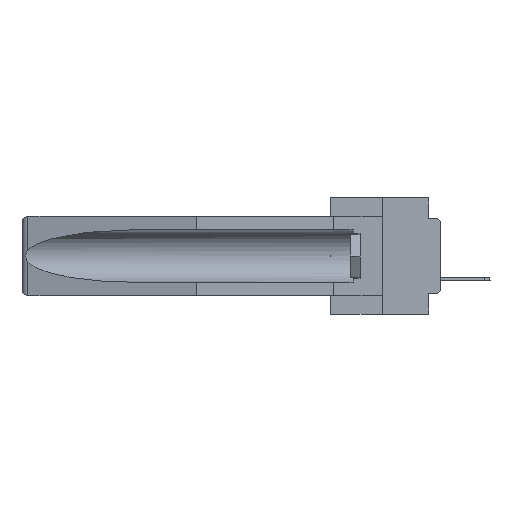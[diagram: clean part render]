
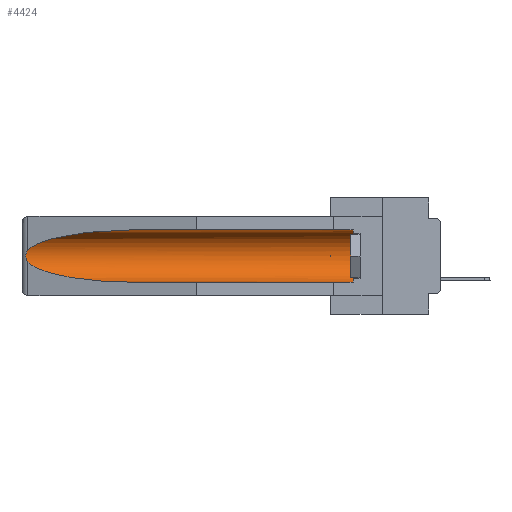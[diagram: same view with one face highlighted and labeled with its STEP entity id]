
A CAD part, left-side view. The second image highlights one B-rep face of the part: STEP entity #4424.
In plain terms, the highlighted cylindrical face has radius 2.857 mm (diameter 5.715 mm), a partial arc.
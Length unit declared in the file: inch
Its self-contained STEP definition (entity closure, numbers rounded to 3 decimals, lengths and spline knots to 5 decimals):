
#463 = EDGE_CURVE ( 'NONE', #9557, #4743, #7884, .T. ) ;
#1396 = CARTESIAN_POINT ( 'NONE',  ( 0.155, -0.30754, -0.284 ) ) ;
#2283 = CARTESIAN_POINT ( 'NONE',  ( 0.2673, 1.53269, -0.17917 ) ) ;
#2791 = DIRECTION ( 'NONE',  ( 0., 1., 0. ) ) ;
#3652 = VECTOR ( 'NONE', #22807, 39.37008 ) ;
#4424 = ADVANCED_FACE ( 'NONE', ( #13636 ), #19963, .F. ) ;
#4743 = VERTEX_POINT ( 'NONE', #22501 ) ;
#5068 = CARTESIAN_POINT ( 'NONE',  ( 0.26654, 1.53092, -0.15636 ) ) ;
#5445 = CIRCLE ( 'NONE', #13716, 0.1125 ) ;
#6375 = EDGE_CURVE ( 'NONE', #7409, #33984, #18339, .T. ) ;
#6435 = CARTESIAN_POINT ( 'NONE',  ( 0.155, 0.126, -0.284 ) ) ;
#7055 = CARTESIAN_POINT ( 'NONE',  ( 0.26537, 1.52718, -0.14972 ) ) ;
#7095 = DIRECTION ( 'NONE',  ( 0., 1., 0. ) ) ;
#7409 = VERTEX_POINT ( 'NONE', #22976 ) ;
#7884 =( BOUNDED_CURVE ( )  B_SPLINE_CURVE ( 3, ( #34929, #10754, #35115, #38264 ),
 .UNSPECIFIED., .F., .F. ) 
 B_SPLINE_CURVE_WITH_KNOTS ( ( 4, 4 ),
 ( 0.1948, 1.5708 ),
 .UNSPECIFIED. ) 
 CURVE ( )  GEOMETRIC_REPRESENTATION_ITEM ( )  RATIONAL_B_SPLINE_CURVE ( ( 1., 0.848, 0.848, 1. ) ) 
 REPRESENTATION_ITEM ( '' )  );
#8369 = CARTESIAN_POINT ( 'NONE',  ( 0.155, -0.30754, -0.059 ) ) ;
#8754 = VECTOR ( 'NONE', #2791, 39.37008 ) ;
#9080 = ORIENTED_EDGE ( 'NONE', *, *, #28041, .T. ) ;
#9557 = VERTEX_POINT ( 'NONE', #36418 ) ;
#10074 = CARTESIAN_POINT ( 'NONE',  ( 0.25451, 1.48313, -0.09465 ) ) ;
#10754 = CARTESIAN_POINT ( 'NONE',  ( 0.25451, 1.48313, -0.24835 ) ) ;
#11154 = EDGE_CURVE ( 'NONE', #33984, #9557, #23094, .T. ) ;
#11438 = CARTESIAN_POINT ( 'NONE',  ( 0.26597, 1.5296, -0.19026 ) ) ;
#12276 = CARTESIAN_POINT ( 'NONE',  ( 0.21114, 1.30732, -0.059 ) ) ;
#13636 = FACE_OUTER_BOUND ( 'NONE', #32733, .T. ) ;
#13716 = AXIS2_PLACEMENT_3D ( 'NONE', #17679, #20637, #29754 ) ;
#15459 = ORIENTED_EDGE ( 'NONE', *, *, #29558, .F. ) ;
#16698 = CARTESIAN_POINT ( 'NONE',  ( 0.155, 0.126, -0.059 ) ) ;
#17679 = CARTESIAN_POINT ( 'NONE',  ( 0.155, 0.126, -0.1715 ) ) ;
#18339 =( BOUNDED_CURVE ( )  B_SPLINE_CURVE ( 3, ( #37214, #12276, #10074, #27896 ),
 .UNSPECIFIED., .F., .F. ) 
 B_SPLINE_CURVE_WITH_KNOTS ( ( 4, 4 ),
 ( 4.71239, 6.08839 ),
 .UNSPECIFIED. ) 
 CURVE ( )  GEOMETRIC_REPRESENTATION_ITEM ( )  RATIONAL_B_SPLINE_CURVE ( ( 1., 0.848, 0.848, 1. ) ) 
 REPRESENTATION_ITEM ( '' )  );
#19208 = CARTESIAN_POINT ( 'NONE',  ( 0.155, -0.30754, -0.1715 ) ) ;
#19449 = LINE ( 'NONE', #1396, #3652 ) ;
#19963 = CYLINDRICAL_SURFACE ( 'NONE', #31102, 0.1125 ) ;
#20637 = DIRECTION ( 'NONE',  ( 0., -1., 0. ) ) ;
#22408 = ORIENTED_EDGE ( 'NONE', *, *, #463, .T. ) ;
#22501 = CARTESIAN_POINT ( 'NONE',  ( 0.155, 1.07973, -0.284 ) ) ;
#22736 = CARTESIAN_POINT ( 'NONE',  ( 0.2675, 1.53308, -0.16763 ) ) ;
#22807 = DIRECTION ( 'NONE',  ( 0., 1., 0. ) ) ;
#22916 = CARTESIAN_POINT ( 'NONE',  ( 0.2673, 1.5327, -0.16383 ) ) ;
#22976 = CARTESIAN_POINT ( 'NONE',  ( 0.155, 1.07973, -0.059 ) ) ;
#23094 = B_SPLINE_CURVE_WITH_KNOTS ( 'NONE', 3,
 ( #26667, #28867, #5068, #22916, #22736, #29448, #2283, #38574, #11438, #34842 ),
 .UNSPECIFIED., .F., .F.,
 ( 4, 2, 2, 2, 4 ),
 ( 0., 0.00029, 0.00058, 0.00087, 0.00117 ),
 .UNSPECIFIED. ) ;
#23297 = VERTEX_POINT ( 'NONE', #6435 ) ;
#25132 = VERTEX_POINT ( 'NONE', #16698 ) ;
#26667 = CARTESIAN_POINT ( 'NONE',  ( 0.26537, 1.52718, -0.14972 ) ) ;
#27896 = CARTESIAN_POINT ( 'NONE',  ( 0.26537, 1.52718, -0.14972 ) ) ;
#28041 = EDGE_CURVE ( 'NONE', #23297, #25132, #5445, .T. ) ;
#28867 = CARTESIAN_POINT ( 'NONE',  ( 0.26597, 1.52961, -0.15275 ) ) ;
#28892 = ORIENTED_EDGE ( 'NONE', *, *, #11154, .T. ) ;
#29448 = CARTESIAN_POINT ( 'NONE',  ( 0.2675, 1.53308, -0.17534 ) ) ;
#29558 = EDGE_CURVE ( 'NONE', #23297, #4743, #19449, .T. ) ;
#29754 = DIRECTION ( 'NONE',  ( 0., 0., 1. ) ) ;
#29768 = EDGE_CURVE ( 'NONE', #25132, #7409, #38688, .T. ) ;
#31102 = AXIS2_PLACEMENT_3D ( 'NONE', #19208, #7095, #31275 ) ;
#31275 = DIRECTION ( 'NONE',  ( 0., 0., 1. ) ) ;
#32733 = EDGE_LOOP ( 'NONE', ( #36746, #28892, #22408, #15459, #9080, #39087 ) ) ;
#33984 = VERTEX_POINT ( 'NONE', #7055 ) ;
#34842 = CARTESIAN_POINT ( 'NONE',  ( 0.26537, 1.52718, -0.19328 ) ) ;
#34929 = CARTESIAN_POINT ( 'NONE',  ( 0.26537, 1.52718, -0.19328 ) ) ;
#35115 = CARTESIAN_POINT ( 'NONE',  ( 0.21114, 1.30732, -0.284 ) ) ;
#36418 = CARTESIAN_POINT ( 'NONE',  ( 0.26537, 1.52718, -0.19328 ) ) ;
#36746 = ORIENTED_EDGE ( 'NONE', *, *, #6375, .T. ) ;
#37214 = CARTESIAN_POINT ( 'NONE',  ( 0.155, 1.07973, -0.059 ) ) ;
#38264 = CARTESIAN_POINT ( 'NONE',  ( 0.155, 1.07973, -0.284 ) ) ;
#38574 = CARTESIAN_POINT ( 'NONE',  ( 0.26655, 1.53094, -0.18657 ) ) ;
#38688 = LINE ( 'NONE', #8369, #8754 ) ;
#39087 = ORIENTED_EDGE ( 'NONE', *, *, #29768, .T. ) ;
